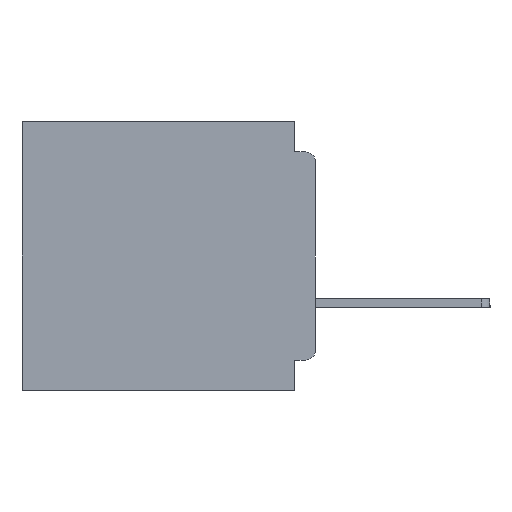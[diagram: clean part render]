
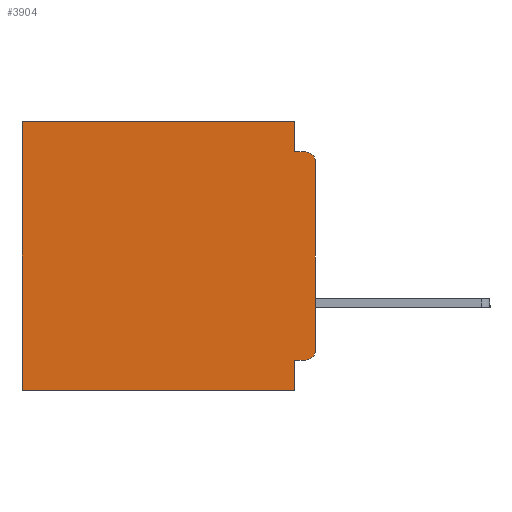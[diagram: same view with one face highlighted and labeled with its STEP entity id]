
A CAD part, left-side view. The second image highlights one B-rep face of the part: STEP entity #3904.
In plain terms, the highlighted planar face has unit normal (-1, 0, 0).
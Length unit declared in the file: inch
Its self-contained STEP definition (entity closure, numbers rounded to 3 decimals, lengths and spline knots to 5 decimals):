
#410 = VERTEX_POINT ( 'NONE', #37167 ) ;
#714 = LINE ( 'NONE', #16472, #33321 ) ;
#1239 = DIRECTION ( 'NONE',  ( 0., 0., -1. ) ) ;
#3602 = CARTESIAN_POINT ( 'NONE',  ( 0.3, 0., -0.4 ) ) ;
#3680 = AXIS2_PLACEMENT_3D ( 'NONE', #31783, #12971, #34935 ) ;
#3681 = VERTEX_POINT ( 'NONE', #16533 ) ;
#3904 = ADVANCED_FACE ( 'NONE', ( #33281 ), #10641, .F. ) ;
#4385 = ORIENTED_EDGE ( 'NONE', *, *, #22250, .T. ) ;
#4745 = DIRECTION ( 'NONE',  ( 0., 0., -1. ) ) ;
#5508 = VECTOR ( 'NONE', #38240, 39.37008 ) ;
#5573 = CARTESIAN_POINT ( 'NONE',  ( 0.3, 0., 0. ) ) ;
#6792 = EDGE_CURVE ( 'NONE', #13247, #33394, #22295, .T. ) ;
#6867 = AXIS2_PLACEMENT_3D ( 'NONE', #27225, #8335, #30383 ) ;
#8005 = CARTESIAN_POINT ( 'NONE',  ( 0.3, 0.031, -0.4 ) ) ;
#8141 = EDGE_CURVE ( 'NONE', #410, #3681, #26621, .T. ) ;
#8262 = VERTEX_POINT ( 'NONE', #11886 ) ;
#8335 = DIRECTION ( 'NONE',  ( -1., 0., 0. ) ) ;
#8868 = VECTOR ( 'NONE', #4745, 39.37008 ) ;
#10164 = LINE ( 'NONE', #16252, #25957 ) ;
#10266 = EDGE_CURVE ( 'NONE', #20357, #24367, #15059, .T. ) ;
#10641 = PLANE ( 'NONE',  #26964 ) ;
#11838 = ORIENTED_EDGE ( 'NONE', *, *, #10266, .F. ) ;
#11886 = CARTESIAN_POINT ( 'NONE',  ( 0.3, 0., -0.34 ) ) ;
#12971 = DIRECTION ( 'NONE',  ( -1., 0., 0. ) ) ;
#13142 = CARTESIAN_POINT ( 'NONE',  ( 0.3, 0., -0.355 ) ) ;
#13247 = VERTEX_POINT ( 'NONE', #32697 ) ;
#13435 = DIRECTION ( 'NONE',  ( 0., 1., 0. ) ) ;
#13897 = VECTOR ( 'NONE', #1239, 39.37008 ) ;
#13913 = ORIENTED_EDGE ( 'NONE', *, *, #8141, .F. ) ;
#13965 = CARTESIAN_POINT ( 'NONE',  ( 0.3, 0.437, -0.4 ) ) ;
#14604 = DIRECTION ( 'NONE',  ( 1., 0., 0. ) ) ;
#14701 = CARTESIAN_POINT ( 'NONE',  ( 0.3, 0.031, 0. ) ) ;
#15059 = LINE ( 'NONE', #36793, #30715 ) ;
#15252 = DIRECTION ( 'NONE',  ( 0., 1., 0. ) ) ;
#16252 = CARTESIAN_POINT ( 'NONE',  ( 0.3, 0., -0.4 ) ) ;
#16472 = CARTESIAN_POINT ( 'NONE',  ( 0.3, 0., -0.4 ) ) ;
#16533 = CARTESIAN_POINT ( 'NONE',  ( 0.3, 0.031, -0.4 ) ) ;
#16733 = EDGE_LOOP ( 'NONE', ( #26308, #37449, #40607, #11838, #4385, #22141, #24975, #13913, #17059, #28045 ) ) ;
#17059 = ORIENTED_EDGE ( 'NONE', *, *, #39491, .F. ) ;
#17741 = EDGE_CURVE ( 'NONE', #24367, #19559, #29873, .T. ) ;
#18031 = DIRECTION ( 'NONE',  ( 0., 0., -1. ) ) ;
#18551 = CIRCLE ( 'NONE', #3680, 0.015 ) ;
#19453 = DIRECTION ( 'NONE',  ( 0., 0., -1. ) ) ;
#19559 = VERTEX_POINT ( 'NONE', #23781 ) ;
#19793 = CARTESIAN_POINT ( 'NONE',  ( 0.3, 0.031, -0.045 ) ) ;
#20357 = VERTEX_POINT ( 'NONE', #14701 ) ;
#20563 = VECTOR ( 'NONE', #32905, 39.37008 ) ;
#22141 = ORIENTED_EDGE ( 'NONE', *, *, #6792, .T. ) ;
#22250 = EDGE_CURVE ( 'NONE', #20357, #13247, #29047, .T. ) ;
#22295 = LINE ( 'NONE', #13965, #13897 ) ;
#23781 = CARTESIAN_POINT ( 'NONE',  ( 0.3, 0.015, -0.045 ) ) ;
#24367 = VERTEX_POINT ( 'NONE', #19793 ) ;
#24411 = VERTEX_POINT ( 'NONE', #29343 ) ;
#24872 = EDGE_CURVE ( 'NONE', #24411, #8262, #18551, .T. ) ;
#24975 = ORIENTED_EDGE ( 'NONE', *, *, #29262, .F. ) ;
#25957 = VECTOR ( 'NONE', #19453, 39.37008 ) ;
#26308 = ORIENTED_EDGE ( 'NONE', *, *, #30347, .F. ) ;
#26621 = LINE ( 'NONE', #8005, #8868 ) ;
#26964 = AXIS2_PLACEMENT_3D ( 'NONE', #3602, #14604, #39319 ) ;
#27078 = VECTOR ( 'NONE', #15252, 39.37008 ) ;
#27225 = CARTESIAN_POINT ( 'NONE',  ( 0.3, 0.015, -0.06 ) ) ;
#28045 = ORIENTED_EDGE ( 'NONE', *, *, #24872, .T. ) ;
#29047 = LINE ( 'NONE', #5573, #27078 ) ;
#29262 = EDGE_CURVE ( 'NONE', #3681, #33394, #714, .T. ) ;
#29343 = CARTESIAN_POINT ( 'NONE',  ( 0.3, 0.015, -0.355 ) ) ;
#29767 = CARTESIAN_POINT ( 'NONE',  ( 0.3, 0., -0.045 ) ) ;
#29873 = LINE ( 'NONE', #29767, #20563 ) ;
#30347 = EDGE_CURVE ( 'NONE', #34556, #8262, #10164, .T. ) ;
#30383 = DIRECTION ( 'NONE',  ( 0., 0., -1. ) ) ;
#30715 = VECTOR ( 'NONE', #18031, 39.37008 ) ;
#31190 = CARTESIAN_POINT ( 'NONE',  ( 0.3, 0.437, -0.4 ) ) ;
#31783 = CARTESIAN_POINT ( 'NONE',  ( 0.3, 0.015, -0.34 ) ) ;
#31869 = CARTESIAN_POINT ( 'NONE',  ( 0.3, 0., -0.06 ) ) ;
#32697 = CARTESIAN_POINT ( 'NONE',  ( 0.3, 0.437, 0. ) ) ;
#32905 = DIRECTION ( 'NONE',  ( 0., -1., 0. ) ) ;
#33230 = EDGE_CURVE ( 'NONE', #34556, #19559, #35180, .T. ) ;
#33281 = FACE_OUTER_BOUND ( 'NONE', #16733, .T. ) ;
#33321 = VECTOR ( 'NONE', #13435, 39.37008 ) ;
#33394 = VERTEX_POINT ( 'NONE', #31190 ) ;
#34556 = VERTEX_POINT ( 'NONE', #31869 ) ;
#34935 = DIRECTION ( 'NONE',  ( 0., 0., -1. ) ) ;
#35180 = CIRCLE ( 'NONE', #6867, 0.015 ) ;
#36793 = CARTESIAN_POINT ( 'NONE',  ( 0.3, 0.031, 0. ) ) ;
#37167 = CARTESIAN_POINT ( 'NONE',  ( 0.3, 0.031, -0.355 ) ) ;
#37449 = ORIENTED_EDGE ( 'NONE', *, *, #33230, .T. ) ;
#38240 = DIRECTION ( 'NONE',  ( 0., 1., 0. ) ) ;
#39044 = LINE ( 'NONE', #13142, #5508 ) ;
#39319 = DIRECTION ( 'NONE',  ( 0., 0., -1. ) ) ;
#39491 = EDGE_CURVE ( 'NONE', #24411, #410, #39044, .T. ) ;
#40607 = ORIENTED_EDGE ( 'NONE', *, *, #17741, .F. ) ;
